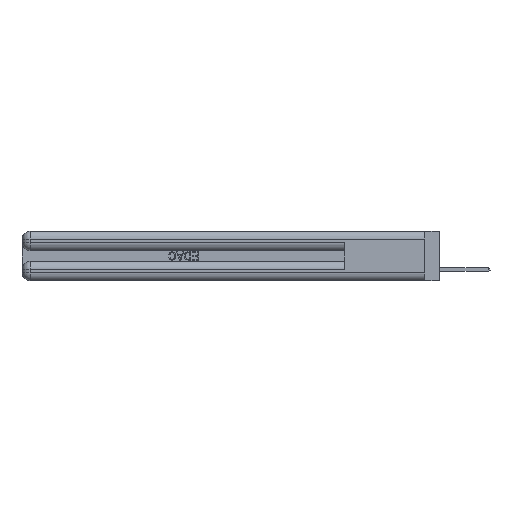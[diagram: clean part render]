
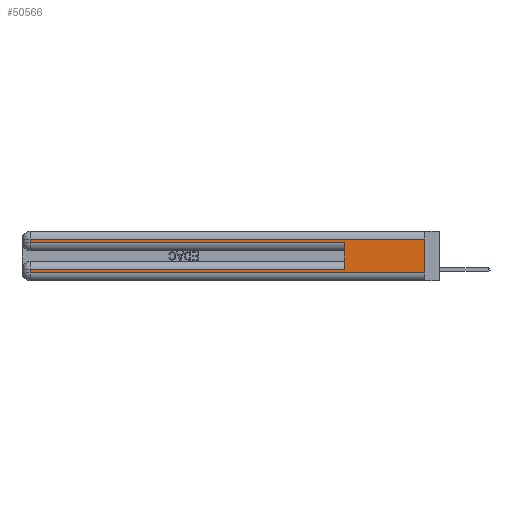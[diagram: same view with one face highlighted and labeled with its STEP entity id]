
A CAD part, left-side view. The second image highlights one B-rep face of the part: STEP entity #50566.
In plain terms, the highlighted planar face has unit normal (-1, 0, 0).
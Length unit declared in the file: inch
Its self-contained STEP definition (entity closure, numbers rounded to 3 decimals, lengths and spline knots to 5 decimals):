
#340 = CARTESIAN_POINT ( 'NONE',  ( 0., 0., 0.085 ) ) ;
#785 = VECTOR ( 'NONE', #44772, 39.37008 ) ;
#1701 = FACE_OUTER_BOUND ( 'NONE', #38852, .T. ) ;
#2254 = ORIENTED_EDGE ( 'NONE', *, *, #25431, .F. ) ;
#3052 = DIRECTION ( 'NONE',  ( 0., 0., -1. ) ) ;
#3103 = VECTOR ( 'NONE', #22174, 39.37008 ) ;
#3399 = CARTESIAN_POINT ( 'NONE',  ( 0., 0., 0.37 ) ) ;
#3545 = ORIENTED_EDGE ( 'NONE', *, *, #42521, .T. ) ;
#3561 = CARTESIAN_POINT ( 'NONE',  ( 0., 2.94, 0.285 ) ) ;
#4939 = CARTESIAN_POINT ( 'NONE',  ( 0., 2.94, 0.37 ) ) ;
#5695 = VECTOR ( 'NONE', #45804, 39.37008 ) ;
#7394 = EDGE_CURVE ( 'NONE', #23834, #35124, #16451, .T. ) ;
#7446 = CARTESIAN_POINT ( 'NONE',  ( 0., 0., 0.06 ) ) ;
#8444 = ORIENTED_EDGE ( 'NONE', *, *, #7394, .T. ) ;
#9574 = EDGE_CURVE ( 'NONE', #24974, #35124, #50679, .T. ) ;
#10132 = PLANE ( 'NONE',  #37684 ) ;
#10491 = CARTESIAN_POINT ( 'NONE',  ( 0., 2.94, 0.37 ) ) ;
#12245 = LINE ( 'NONE', #340, #17818 ) ;
#12728 = ORIENTED_EDGE ( 'NONE', *, *, #43786, .T. ) ;
#12789 = DIRECTION ( 'NONE',  ( 0., 1., 0. ) ) ;
#14312 = CARTESIAN_POINT ( 'NONE',  ( 0., 0., 0.285 ) ) ;
#15345 = DIRECTION ( 'NONE',  ( 0., 0., 1. ) ) ;
#16451 = LINE ( 'NONE', #44443, #785 ) ;
#17573 = CARTESIAN_POINT ( 'NONE',  ( 0., 0., 0.31 ) ) ;
#17818 = VECTOR ( 'NONE', #12789, 39.37008 ) ;
#18039 = VERTEX_POINT ( 'NONE', #49264 ) ;
#19283 = CARTESIAN_POINT ( 'NONE',  ( 0., 2.94, 0.085 ) ) ;
#19329 = CARTESIAN_POINT ( 'NONE',  ( 0., 0.6, 0.145 ) ) ;
#19351 = CARTESIAN_POINT ( 'NONE',  ( 0., 2.94, 0.06 ) ) ;
#20651 = LINE ( 'NONE', #4939, #5695 ) ;
#21751 = VECTOR ( 'NONE', #45327, 39.37008 ) ;
#22024 = CARTESIAN_POINT ( 'NONE',  ( 0., 0., 0.31 ) ) ;
#22171 = DIRECTION ( 'NONE',  ( 1., 0., 0. ) ) ;
#22174 = DIRECTION ( 'NONE',  ( 0., 0., -1. ) ) ;
#22341 = DIRECTION ( 'NONE',  ( 0., -1., 0. ) ) ;
#22528 = VERTEX_POINT ( 'NONE', #3561 ) ;
#23834 = VERTEX_POINT ( 'NONE', #19351 ) ;
#24028 = VERTEX_POINT ( 'NONE', #19283 ) ;
#24471 = EDGE_CURVE ( 'NONE', #47247, #24028, #12245, .T. ) ;
#24974 = VERTEX_POINT ( 'NONE', #22024 ) ;
#25431 = EDGE_CURVE ( 'NONE', #47247, #41059, #51471, .T. ) ;
#25712 = ORIENTED_EDGE ( 'NONE', *, *, #45247, .T. ) ;
#26470 = VECTOR ( 'NONE', #15345, 39.37008 ) ;
#28263 = ORIENTED_EDGE ( 'NONE', *, *, #9574, .F. ) ;
#30027 = ORIENTED_EDGE ( 'NONE', *, *, #38823, .T. ) ;
#32376 = LINE ( 'NONE', #17573, #21751 ) ;
#32428 = LINE ( 'NONE', #10491, #3103 ) ;
#35124 = VERTEX_POINT ( 'NONE', #7446 ) ;
#36311 = ORIENTED_EDGE ( 'NONE', *, *, #24471, .T. ) ;
#37684 = AXIS2_PLACEMENT_3D ( 'NONE', #42574, #22171, #46239 ) ;
#38823 = EDGE_CURVE ( 'NONE', #18039, #22528, #32428, .T. ) ;
#38852 = EDGE_LOOP ( 'NONE', ( #28263, #12728, #30027, #25712, #2254, #36311, #3545, #8444 ) ) ;
#39749 = VECTOR ( 'NONE', #22341, 39.37008 ) ;
#41059 = VERTEX_POINT ( 'NONE', #44954 ) ;
#42521 = EDGE_CURVE ( 'NONE', #24028, #23834, #20651, .T. ) ;
#42574 = CARTESIAN_POINT ( 'NONE',  ( 0., 0., 0.37 ) ) ;
#43786 = EDGE_CURVE ( 'NONE', #24974, #18039, #32376, .T. ) ;
#44443 = CARTESIAN_POINT ( 'NONE',  ( 0., 0., 0.06 ) ) ;
#44772 = DIRECTION ( 'NONE',  ( 0., -1., 0. ) ) ;
#44954 = CARTESIAN_POINT ( 'NONE',  ( 0., 0.6, 0.285 ) ) ;
#45247 = EDGE_CURVE ( 'NONE', #22528, #41059, #46583, .T. ) ;
#45327 = DIRECTION ( 'NONE',  ( 0., 1., 0. ) ) ;
#45804 = DIRECTION ( 'NONE',  ( 0., 0., -1. ) ) ;
#46239 = DIRECTION ( 'NONE',  ( 0., 0., -1. ) ) ;
#46255 = CARTESIAN_POINT ( 'NONE',  ( 0., 0.6, 0.085 ) ) ;
#46583 = LINE ( 'NONE', #14312, #39749 ) ;
#47247 = VERTEX_POINT ( 'NONE', #46255 ) ;
#49264 = CARTESIAN_POINT ( 'NONE',  ( 0., 2.94, 0.31 ) ) ;
#49389 = VECTOR ( 'NONE', #3052, 39.37008 ) ;
#50566 = ADVANCED_FACE ( 'NONE', ( #1701 ), #10132, .F. ) ;
#50679 = LINE ( 'NONE', #3399, #49389 ) ;
#51471 = LINE ( 'NONE', #19329, #26470 ) ;
